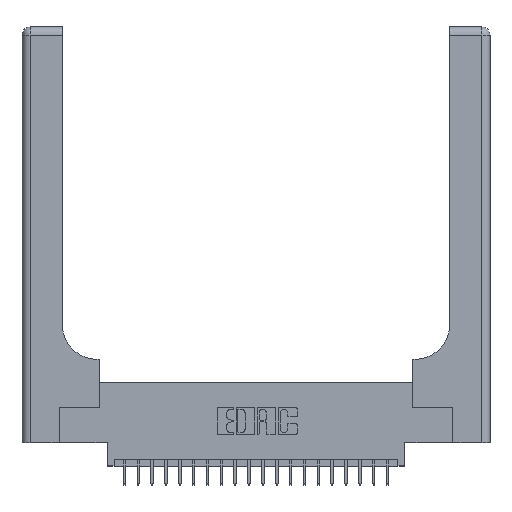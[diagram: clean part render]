
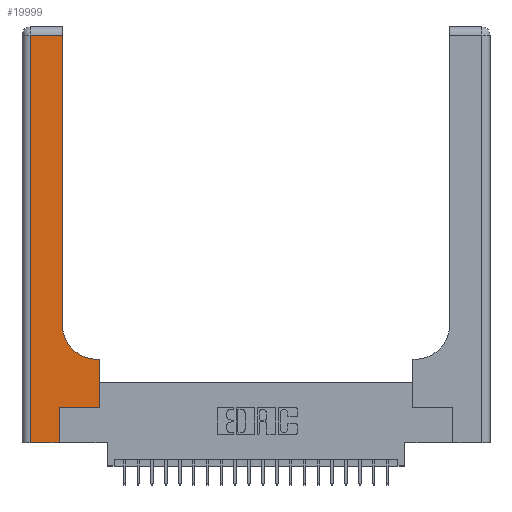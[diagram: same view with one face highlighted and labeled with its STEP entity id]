
A CAD part, top view. The second image highlights one B-rep face of the part: STEP entity #19999.
In plain terms, the highlighted planar face has unit normal (0, 0, 1).
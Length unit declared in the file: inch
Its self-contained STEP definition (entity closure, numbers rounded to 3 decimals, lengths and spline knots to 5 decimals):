
#230 = CARTESIAN_POINT ( 'NONE',  ( 0.269, 0., 0.37 ) ) ;
#235 = VERTEX_POINT ( 'NONE', #3448 ) ;
#354 = ORIENTED_EDGE ( 'NONE', *, *, #2895, .T. ) ;
#408 = DIRECTION ( 'NONE',  ( -1., 0., 0. ) ) ;
#440 = LINE ( 'NONE', #22742, #13214 ) ;
#1222 = EDGE_CURVE ( 'NONE', #6481, #4202, #1376, .T. ) ;
#1348 = VERTEX_POINT ( 'NONE', #4640 ) ;
#1376 = LINE ( 'NONE', #16414, #6018 ) ;
#1558 = VECTOR ( 'NONE', #408, 39.37008 ) ;
#1572 = CARTESIAN_POINT ( 'NONE',  ( 0.2915, 3., 0.37 ) ) ;
#1626 = DIRECTION ( 'NONE',  ( 0., 0., -1. ) ) ;
#2148 = CARTESIAN_POINT ( 'NONE',  ( 0.269, 0., 0.37 ) ) ;
#2191 = VERTEX_POINT ( 'NONE', #12539 ) ;
#2895 = EDGE_CURVE ( 'NONE', #235, #20612, #12032, .T. ) ;
#3448 = CARTESIAN_POINT ( 'NONE',  ( 0.06, 2.94, 0.37 ) ) ;
#3792 = ORIENTED_EDGE ( 'NONE', *, *, #7179, .T. ) ;
#4202 = VERTEX_POINT ( 'NONE', #7589 ) ;
#4640 = CARTESIAN_POINT ( 'NONE',  ( 0.269, 0.25, 0.37 ) ) ;
#4714 = CARTESIAN_POINT ( 'NONE',  ( 0.269, 0.25, 0.37 ) ) ;
#4806 = DIRECTION ( 'NONE',  ( 0., -1., 0. ) ) ;
#4877 = CARTESIAN_POINT ( 'NONE',  ( 0.5585, 0.25, 0.37 ) ) ;
#5016 = ORIENTED_EDGE ( 'NONE', *, *, #15277, .T. ) ;
#5076 = DIRECTION ( 'NONE',  ( 1., 0., 0. ) ) ;
#5163 = DIRECTION ( 'NONE',  ( -1., 0., 0. ) ) ;
#5943 = DIRECTION ( 'NONE',  ( 0., 0., -1. ) ) ;
#6018 = VECTOR ( 'NONE', #23817, 39.37008 ) ;
#6027 = CARTESIAN_POINT ( 'NONE',  ( 0.2915, 2.94, 0.37 ) ) ;
#6030 = EDGE_CURVE ( 'NONE', #6412, #235, #440, .T. ) ;
#6065 = AXIS2_PLACEMENT_3D ( 'NONE', #9065, #1626, #5163 ) ;
#6412 = VERTEX_POINT ( 'NONE', #6027 ) ;
#6481 = VERTEX_POINT ( 'NONE', #4877 ) ;
#6614 = AXIS2_PLACEMENT_3D ( 'NONE', #15236, #5943, #17190 ) ;
#6886 = VERTEX_POINT ( 'NONE', #10687 ) ;
#7100 = ORIENTED_EDGE ( 'NONE', *, *, #22076, .T. ) ;
#7179 = EDGE_CURVE ( 'NONE', #6886, #2191, #15984, .T. ) ;
#7444 = ORIENTED_EDGE ( 'NONE', *, *, #17494, .T. ) ;
#7589 = CARTESIAN_POINT ( 'NONE',  ( 0.5585, 0.6, 0.37 ) ) ;
#8058 = VECTOR ( 'NONE', #24014, 39.37008 ) ;
#8631 = DIRECTION ( 'NONE',  ( 1., 0., 0. ) ) ;
#8989 = VECTOR ( 'NONE', #15244, 39.37008 ) ;
#9065 = CARTESIAN_POINT ( 'NONE',  ( 0., 3., 0.37 ) ) ;
#9383 = EDGE_LOOP ( 'NONE', ( #19921, #10727, #354, #5016, #7100, #7444, #20030, #15191, #3792 ) ) ;
#10090 = CARTESIAN_POINT ( 'NONE',  ( 0.06, 0., 0.37 ) ) ;
#10687 = CARTESIAN_POINT ( 'NONE',  ( 0.5415, 0.6, 0.37 ) ) ;
#10727 = ORIENTED_EDGE ( 'NONE', *, *, #6030, .T. ) ;
#11419 = VERTEX_POINT ( 'NONE', #2148 ) ;
#11955 = CARTESIAN_POINT ( 'NONE',  ( 0.2915, 0.6, 0.37 ) ) ;
#12032 = LINE ( 'NONE', #17427, #12603 ) ;
#12539 = CARTESIAN_POINT ( 'NONE',  ( 0.2915, 0.85, 0.37 ) ) ;
#12603 = VECTOR ( 'NONE', #4806, 39.37008 ) ;
#12836 = VECTOR ( 'NONE', #8631, 39.37008 ) ;
#13214 = VECTOR ( 'NONE', #13835, 39.37008 ) ;
#13287 = VECTOR ( 'NONE', #5076, 39.37008 ) ;
#13835 = DIRECTION ( 'NONE',  ( -1., 0., 0. ) ) ;
#13895 = LINE ( 'NONE', #17925, #12836 ) ;
#14456 = FACE_OUTER_BOUND ( 'NONE', #9383, .T. ) ;
#15191 = ORIENTED_EDGE ( 'NONE', *, *, #16961, .T. ) ;
#15236 = CARTESIAN_POINT ( 'NONE',  ( 0.5415, 0.85, 0.37 ) ) ;
#15244 = DIRECTION ( 'NONE',  ( 0., 1., 0. ) ) ;
#15277 = EDGE_CURVE ( 'NONE', #20612, #11419, #13895, .T. ) ;
#15765 = LINE ( 'NONE', #11955, #1558 ) ;
#15969 = LINE ( 'NONE', #4714, #13287 ) ;
#15984 = CIRCLE ( 'NONE', #6614, 0.25 ) ;
#16414 = CARTESIAN_POINT ( 'NONE',  ( 0.5585, 0.25, 0.37 ) ) ;
#16961 = EDGE_CURVE ( 'NONE', #4202, #6886, #15765, .T. ) ;
#17190 = DIRECTION ( 'NONE',  ( 1., 0., 0. ) ) ;
#17427 = CARTESIAN_POINT ( 'NONE',  ( 0.06, 3., 0.37 ) ) ;
#17494 = EDGE_CURVE ( 'NONE', #1348, #6481, #15969, .T. ) ;
#17925 = CARTESIAN_POINT ( 'NONE',  ( 0., 0., 0.37 ) ) ;
#18431 = LINE ( 'NONE', #1572, #8058 ) ;
#18640 = LINE ( 'NONE', #230, #8989 ) ;
#19921 = ORIENTED_EDGE ( 'NONE', *, *, #20248, .T. ) ;
#19999 = ADVANCED_FACE ( 'NONE', ( #14456 ), #21890, .F. ) ;
#20030 = ORIENTED_EDGE ( 'NONE', *, *, #1222, .T. ) ;
#20248 = EDGE_CURVE ( 'NONE', #2191, #6412, #18431, .T. ) ;
#20612 = VERTEX_POINT ( 'NONE', #10090 ) ;
#21890 = PLANE ( 'NONE',  #6065 ) ;
#22076 = EDGE_CURVE ( 'NONE', #11419, #1348, #18640, .T. ) ;
#22742 = CARTESIAN_POINT ( 'NONE',  ( 0., 2.94, 0.37 ) ) ;
#23817 = DIRECTION ( 'NONE',  ( 0., 1., 0. ) ) ;
#24014 = DIRECTION ( 'NONE',  ( 0., 1., 0. ) ) ;
